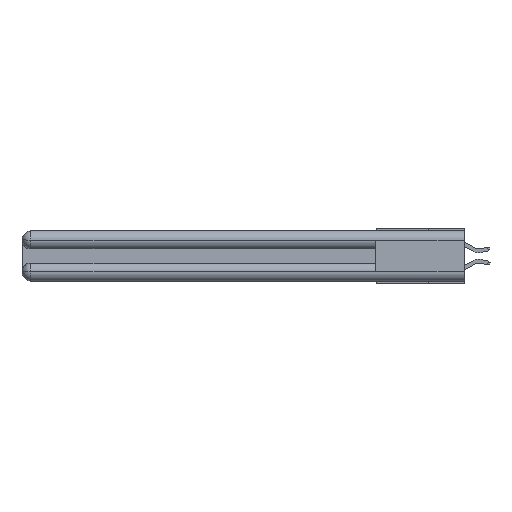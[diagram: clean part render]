
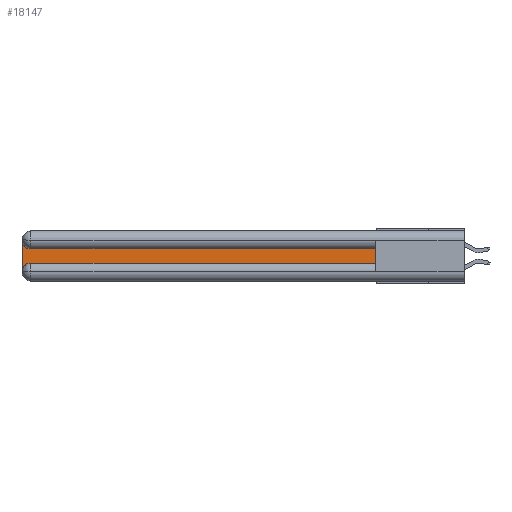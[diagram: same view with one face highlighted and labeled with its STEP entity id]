
A CAD part, left-side view. The second image highlights one B-rep face of the part: STEP entity #18147.
In plain terms, the highlighted planar face has unit normal (-1, 0, 0).
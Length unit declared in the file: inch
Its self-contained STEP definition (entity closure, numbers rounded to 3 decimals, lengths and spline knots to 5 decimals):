
#441 = EDGE_CURVE ( 'NONE', #3616, #22397, #23483, .T. ) ;
#916 = ORIENTED_EDGE ( 'NONE', *, *, #5859, .T. ) ;
#2501 = ORIENTED_EDGE ( 'NONE', *, *, #9977, .T. ) ;
#2561 = CARTESIAN_POINT ( 'NONE',  ( 0.075, 3., -0.1225 ) ) ;
#2829 = CARTESIAN_POINT ( 'NONE',  ( 0.075, 3., -0.0625 ) ) ;
#3221 = CARTESIAN_POINT ( 'NONE',  ( 0.075, 3., -0.2775 ) ) ;
#3283 = ORIENTED_EDGE ( 'NONE', *, *, #9682, .T. ) ;
#3504 = VERTEX_POINT ( 'NONE', #14588 ) ;
#3616 = VERTEX_POINT ( 'NONE', #10321 ) ;
#3834 = VECTOR ( 'NONE', #23312, 39.37008 ) ;
#4167 = VERTEX_POINT ( 'NONE', #12955 ) ;
#4733 = AXIS2_PLACEMENT_3D ( 'NONE', #19708, #6987, #24012 ) ;
#4971 = DIRECTION ( 'NONE',  ( 0., 0., -1. ) ) ;
#5741 = VERTEX_POINT ( 'NONE', #22145 ) ;
#5859 = EDGE_CURVE ( 'NONE', #5741, #3616, #14227, .T. ) ;
#6987 = DIRECTION ( 'NONE',  ( 1., 0., 0. ) ) ;
#7815 = LINE ( 'NONE', #10801, #3834 ) ;
#8061 = EDGE_CURVE ( 'NONE', #22397, #23838, #7815, .T. ) ;
#8385 = FACE_OUTER_BOUND ( 'NONE', #24046, .T. ) ;
#9335 = CARTESIAN_POINT ( 'NONE',  ( 0.075, 2.94, -0.0625 ) ) ;
#9682 = EDGE_CURVE ( 'NONE', #3504, #4167, #10056, .T. ) ;
#9977 = EDGE_CURVE ( 'NONE', #23838, #3504, #12985, .T. ) ;
#10056 = LINE ( 'NONE', #17150, #20719 ) ;
#10321 = CARTESIAN_POINT ( 'NONE',  ( 0.075, 2.94, -0.1225 ) ) ;
#10801 = CARTESIAN_POINT ( 'NONE',  ( 0.075, 3., -0.2175 ) ) ;
#12167 = CARTESIAN_POINT ( 'NONE',  ( 0.075, 0.6, -0.2175 ) ) ;
#12955 = CARTESIAN_POINT ( 'NONE',  ( 0.075, 0.6, -0.2175 ) ) ;
#12985 = CIRCLE ( 'NONE', #4733, 0.06 ) ;
#13073 = DIRECTION ( 'NONE',  ( 1., 0., 0. ) ) ;
#13602 = DIRECTION ( 'NONE',  ( 0., 1., 0. ) ) ;
#14227 = LINE ( 'NONE', #22206, #20245 ) ;
#14588 = CARTESIAN_POINT ( 'NONE',  ( 0.075, 2.94, -0.2175 ) ) ;
#16476 = VECTOR ( 'NONE', #27138, 39.37008 ) ;
#16690 = EDGE_CURVE ( 'NONE', #4167, #5741, #22142, .T. ) ;
#17150 = CARTESIAN_POINT ( 'NONE',  ( 0.075, 0.6, -0.2175 ) ) ;
#17263 = ORIENTED_EDGE ( 'NONE', *, *, #441, .T. ) ;
#18147 = ADVANCED_FACE ( 'NONE', ( #8385 ), #19229, .F. ) ;
#19002 = ORIENTED_EDGE ( 'NONE', *, *, #8061, .T. ) ;
#19183 = AXIS2_PLACEMENT_3D ( 'NONE', #9335, #26402, #4971 ) ;
#19229 = PLANE ( 'NONE',  #21434 ) ;
#19708 = CARTESIAN_POINT ( 'NONE',  ( 0.075, 2.94, -0.2775 ) ) ;
#20183 = ORIENTED_EDGE ( 'NONE', *, *, #16690, .T. ) ;
#20245 = VECTOR ( 'NONE', #13602, 39.37008 ) ;
#20719 = VECTOR ( 'NONE', #26052, 39.37008 ) ;
#21434 = AXIS2_PLACEMENT_3D ( 'NONE', #2561, #13073, #26059 ) ;
#22142 = LINE ( 'NONE', #12167, #16476 ) ;
#22145 = CARTESIAN_POINT ( 'NONE',  ( 0.075, 0.6, -0.1225 ) ) ;
#22206 = CARTESIAN_POINT ( 'NONE',  ( 0.075, 0.6, -0.1225 ) ) ;
#22397 = VERTEX_POINT ( 'NONE', #2829 ) ;
#23312 = DIRECTION ( 'NONE',  ( 0., 0., -1. ) ) ;
#23483 = CIRCLE ( 'NONE', #19183, 0.06 ) ;
#23838 = VERTEX_POINT ( 'NONE', #3221 ) ;
#24012 = DIRECTION ( 'NONE',  ( 0., 0., -1. ) ) ;
#24046 = EDGE_LOOP ( 'NONE', ( #916, #17263, #19002, #2501, #3283, #20183 ) ) ;
#26052 = DIRECTION ( 'NONE',  ( 0., -1., 0. ) ) ;
#26059 = DIRECTION ( 'NONE',  ( 0., 0., -1. ) ) ;
#26402 = DIRECTION ( 'NONE',  ( 1., 0., 0. ) ) ;
#27138 = DIRECTION ( 'NONE',  ( 0., 0., 1. ) ) ;
